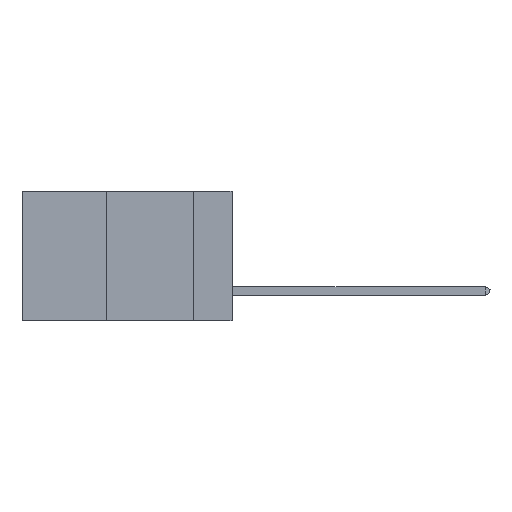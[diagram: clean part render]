
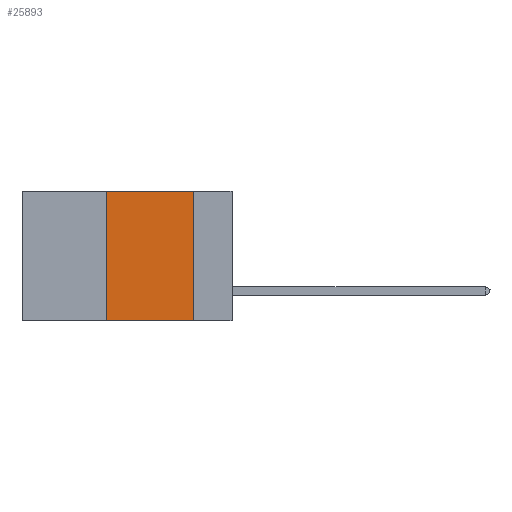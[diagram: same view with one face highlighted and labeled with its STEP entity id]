
A CAD part, left-side view. The second image highlights one B-rep face of the part: STEP entity #25893.
In plain terms, the highlighted planar face has unit normal (-1, 0, 0).
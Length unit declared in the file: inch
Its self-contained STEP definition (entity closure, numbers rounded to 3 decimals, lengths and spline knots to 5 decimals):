
#392 = DIRECTION ( 'NONE',  ( 0., -1., 0. ) ) ;
#562 = DIRECTION ( 'NONE',  ( 0., -1., 0. ) ) ;
#1313 = DIRECTION ( 'NONE',  ( 0., 0., 1. ) ) ;
#2624 = VECTOR ( 'NONE', #1313, 39.37008 ) ;
#3523 = CARTESIAN_POINT ( 'NONE',  ( 0., 0.6, 0. ) ) ;
#3931 = CARTESIAN_POINT ( 'NONE',  ( 0., 0.6, -0.37 ) ) ;
#3932 = CARTESIAN_POINT ( 'NONE',  ( 0., 0.36, -0.37 ) ) ;
#7205 = LINE ( 'NONE', #3523, #26266 ) ;
#8380 = EDGE_CURVE ( 'NONE', #9665, #29833, #8444, .T. ) ;
#8400 = DIRECTION ( 'NONE',  ( 0., 0., -1. ) ) ;
#8444 = LINE ( 'NONE', #29784, #26940 ) ;
#9665 = VERTEX_POINT ( 'NONE', #41317 ) ;
#10527 = VERTEX_POINT ( 'NONE', #3932 ) ;
#11698 = PLANE ( 'NONE',  #25133 ) ;
#12087 = ORIENTED_EDGE ( 'NONE', *, *, #31021, .F. ) ;
#13687 = EDGE_LOOP ( 'NONE', ( #39638, #12087, #20562, #22876 ) ) ;
#14386 = VERTEX_POINT ( 'NONE', #29097 ) ;
#16811 = EDGE_CURVE ( 'NONE', #10527, #14386, #17086, .T. ) ;
#17086 = LINE ( 'NONE', #22072, #2624 ) ;
#20562 = ORIENTED_EDGE ( 'NONE', *, *, #16811, .F. ) ;
#21135 = CARTESIAN_POINT ( 'NONE',  ( 0., 0.6, 0. ) ) ;
#22072 = CARTESIAN_POINT ( 'NONE',  ( 0., 0.36, 0. ) ) ;
#22412 = LINE ( 'NONE', #3931, #33396 ) ;
#22876 = ORIENTED_EDGE ( 'NONE', *, *, #29922, .T. ) ;
#24694 = DIRECTION ( 'NONE',  ( 1., 0., 0. ) ) ;
#25133 = AXIS2_PLACEMENT_3D ( 'NONE', #21135, #24694, #8400 ) ;
#25893 = ADVANCED_FACE ( 'NONE', ( #39815 ), #11698, .F. ) ;
#25923 = CARTESIAN_POINT ( 'NONE',  ( 0., 0.11, -0.37 ) ) ;
#26266 = VECTOR ( 'NONE', #392, 39.37008 ) ;
#26940 = VECTOR ( 'NONE', #39731, 39.37008 ) ;
#29097 = CARTESIAN_POINT ( 'NONE',  ( 0., 0.36, 0. ) ) ;
#29784 = CARTESIAN_POINT ( 'NONE',  ( 0., 0.11, 0. ) ) ;
#29833 = VERTEX_POINT ( 'NONE', #25923 ) ;
#29922 = EDGE_CURVE ( 'NONE', #10527, #29833, #22412, .T. ) ;
#31021 = EDGE_CURVE ( 'NONE', #14386, #9665, #7205, .T. ) ;
#33396 = VECTOR ( 'NONE', #562, 39.37008 ) ;
#39638 = ORIENTED_EDGE ( 'NONE', *, *, #8380, .F. ) ;
#39731 = DIRECTION ( 'NONE',  ( 0., 0., -1. ) ) ;
#39815 = FACE_OUTER_BOUND ( 'NONE', #13687, .T. ) ;
#41317 = CARTESIAN_POINT ( 'NONE',  ( 0., 0.11, 0. ) ) ;
